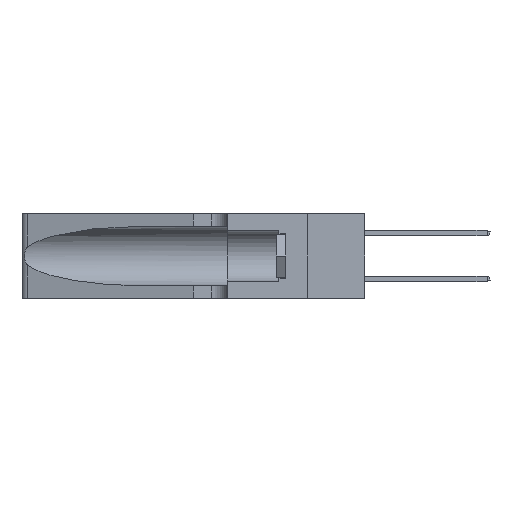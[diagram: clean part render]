
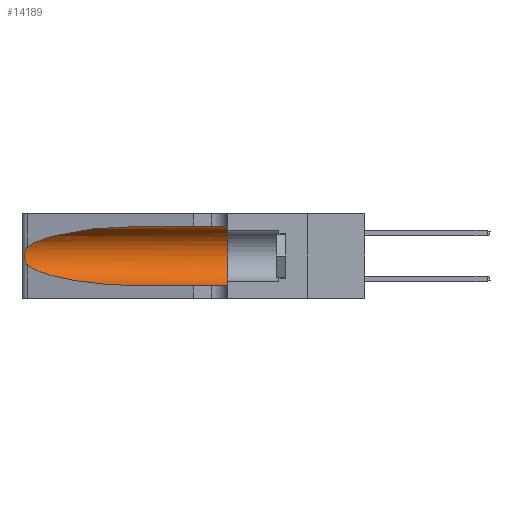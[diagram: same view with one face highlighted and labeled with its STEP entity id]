
A CAD part, left-side view. The second image highlights one B-rep face of the part: STEP entity #14189.
In plain terms, the highlighted cylindrical face has radius 3.308 mm (diameter 6.617 mm), a partial arc.
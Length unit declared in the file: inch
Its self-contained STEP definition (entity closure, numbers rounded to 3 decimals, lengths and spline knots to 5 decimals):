
#309 = CARTESIAN_POINT ( 'NONE',  ( 0.26075, 1.23896, 0.178 ) ) ;
#966 = EDGE_CURVE ( 'NONE', #5976, #19611, #1020, .T. ) ;
#1020 = LINE ( 'NONE', #4314, #5812 ) ;
#2368 = CARTESIAN_POINT ( 'NONE',  ( 0.25856, 1.23593, 0.16098 ) ) ;
#4084 = DIRECTION ( 'NONE',  ( 0., -1., 0. ) ) ;
#4173 = CARTESIAN_POINT ( 'NONE',  ( 0.25487, 1.22718, 0.22369 ) ) ;
#4314 = CARTESIAN_POINT ( 'NONE',  ( 0.1305, 1.61858, 0.05475 ) ) ;
#4342 = CARTESIAN_POINT ( 'NONE',  ( 0.25639, 1.23184, 0.21858 ) ) ;
#4435 = CARTESIAN_POINT ( 'NONE',  ( 0.25639, 1.23186, 0.15144 ) ) ;
#4637 = ORIENTED_EDGE ( 'NONE', *, *, #966, .T. ) ;
#4742 = CYLINDRICAL_SURFACE ( 'NONE', #22017, 0.13025 ) ;
#4822 = CARTESIAN_POINT ( 'NONE',  ( 0.18966, 0.96281, 0.05475 ) ) ;
#4998 = CARTESIAN_POINT ( 'NONE',  ( 0.1305, 0.35, 0.05475 ) ) ;
#5384 = EDGE_CURVE ( 'NONE', #10607, #19153, #17076, .T. ) ;
#5812 = VECTOR ( 'NONE', #4084, 39.37008 ) ;
#5912 = DIRECTION ( 'NONE',  ( 0., 0., -1. ) ) ;
#5976 = VERTEX_POINT ( 'NONE', #10400 ) ;
#6082 = AXIS2_PLACEMENT_3D ( 'NONE', #10811, #24309, #12737 ) ;
#6107 = CARTESIAN_POINT ( 'NONE',  ( 0.18966, 0.96281, 0.31525 ) ) ;
#6442 = CARTESIAN_POINT ( 'NONE',  ( 0.25487, 1.22718, 0.14631 ) ) ;
#6706 = CIRCLE ( 'NONE', #6082, 0.13025 ) ;
#6737 = CARTESIAN_POINT ( 'NONE',  ( 0.25487, 1.22718, 0.14631 ) ) ;
#8091 = VERTEX_POINT ( 'NONE', #13316 ) ;
#8113 = CARTESIAN_POINT ( 'NONE',  ( 0.1305, 0.72297, 0.31525 ) ) ;
#8356 = CARTESIAN_POINT ( 'NONE',  ( 0.25487, 1.22718, 0.22369 ) ) ;
#8822 = CARTESIAN_POINT ( 'NONE',  ( 0.25487, 1.22718, 0.22369 ) ) ;
#9886 = CARTESIAN_POINT ( 'NONE',  ( 0.1305, 1.61858, 0.185 ) ) ;
#10324 = CARTESIAN_POINT ( 'NONE',  ( 0.25854, 1.2359, 0.20912 ) ) ;
#10400 = CARTESIAN_POINT ( 'NONE',  ( 0.1305, 0.72297, 0.05475 ) ) ;
#10607 = VERTEX_POINT ( 'NONE', #8822 ) ;
#10729 =( BOUNDED_CURVE ( )  B_SPLINE_CURVE ( 3, ( #6737, #14575, #4822, #18486 ),
 .UNSPECIFIED., .F., .F. ) 
 B_SPLINE_CURVE_WITH_KNOTS ( ( 4, 4 ),
 ( 3.44316, 4.71239 ),
 .UNSPECIFIED. ) 
 CURVE ( )  GEOMETRIC_REPRESENTATION_ITEM ( )  RATIONAL_B_SPLINE_CURVE ( ( 1., 0.87, 0.87, 1. ) ) 
 REPRESENTATION_ITEM ( '' )  );
#10811 = CARTESIAN_POINT ( 'NONE',  ( 0.1305, 0.35, 0.185 ) ) ;
#10864 = VERTEX_POINT ( 'NONE', #19232 ) ;
#12256 = CARTESIAN_POINT ( 'NONE',  ( 0.26075, 1.23896, 0.19203 ) ) ;
#12737 = DIRECTION ( 'NONE',  ( 0., 0., 1. ) ) ;
#13316 = CARTESIAN_POINT ( 'NONE',  ( 0.1305, 0.72297, 0.31525 ) ) ;
#13585 = EDGE_CURVE ( 'NONE', #8091, #10607, #15205, .T. ) ;
#14188 = CARTESIAN_POINT ( 'NONE',  ( 0.26017, 1.23833, 0.17102 ) ) ;
#14189 = ADVANCED_FACE ( 'NONE', ( #20273 ), #4742, .F. ) ;
#14575 = CARTESIAN_POINT ( 'NONE',  ( 0.2373, 1.15595, 0.08982 ) ) ;
#14754 = CARTESIAN_POINT ( 'NONE',  ( 0.1305, 1.61858, 0.31525 ) ) ;
#15110 = EDGE_CURVE ( 'NONE', #19153, #5976, #10729, .T. ) ;
#15205 =( BOUNDED_CURVE ( )  B_SPLINE_CURVE ( 3, ( #8113, #6107, #15912, #4173 ),
 .UNSPECIFIED., .F., .T. ) 
 B_SPLINE_CURVE_WITH_KNOTS ( ( 4, 4 ),
 ( 1.5708, 2.84003 ),
 .UNSPECIFIED. ) 
 CURVE ( )  GEOMETRIC_REPRESENTATION_ITEM ( )  RATIONAL_B_SPLINE_CURVE ( ( 1., 0.87, 0.87, 1. ) ) 
 REPRESENTATION_ITEM ( '' )  );
#15912 = CARTESIAN_POINT ( 'NONE',  ( 0.2373, 1.15595, 0.28018 ) ) ;
#16100 = VECTOR ( 'NONE', #20565, 39.37008 ) ;
#16155 = CARTESIAN_POINT ( 'NONE',  ( 0.25789, 1.23486, 0.15765 ) ) ;
#17076 = B_SPLINE_CURVE_WITH_KNOTS ( 'NONE', 3,
 ( #8356, #18014, #4342, #21874, #10324, #23808, #12256, #309, #14188, #2368, #16155, #4435, #18101, #6442 ),
 .UNSPECIFIED., .F., .F.,
 ( 4, 2, 2, 2, 2, 2, 4 ),
 ( 0., 0.00027, 0.00053, 0.00107, 0.0016, 0.00187, 0.00214 ),
 .UNSPECIFIED. ) ;
#17082 = ORIENTED_EDGE ( 'NONE', *, *, #13585, .T. ) ;
#18014 = CARTESIAN_POINT ( 'NONE',  ( 0.25555, 1.22994, 0.2215 ) ) ;
#18027 = CARTESIAN_POINT ( 'NONE',  ( 0.25487, 1.22718, 0.14631 ) ) ;
#18101 = CARTESIAN_POINT ( 'NONE',  ( 0.25555, 1.22993, 0.14849 ) ) ;
#18486 = CARTESIAN_POINT ( 'NONE',  ( 0.1305, 0.72297, 0.05475 ) ) ;
#19153 = VERTEX_POINT ( 'NONE', #18027 ) ;
#19232 = CARTESIAN_POINT ( 'NONE',  ( 0.1305, 0.35, 0.31525 ) ) ;
#19575 = ORIENTED_EDGE ( 'NONE', *, *, #15110, .T. ) ;
#19611 = VERTEX_POINT ( 'NONE', #4998 ) ;
#19620 = EDGE_CURVE ( 'NONE', #8091, #10864, #21821, .T. ) ;
#20273 = FACE_OUTER_BOUND ( 'NONE', #21672, .T. ) ;
#20565 = DIRECTION ( 'NONE',  ( 0., -1., 0. ) ) ;
#20867 = EDGE_CURVE ( 'NONE', #10864, #19611, #6706, .T. ) ;
#20894 = ORIENTED_EDGE ( 'NONE', *, *, #19620, .F. ) ;
#21518 = ORIENTED_EDGE ( 'NONE', *, *, #20867, .F. ) ;
#21672 = EDGE_LOOP ( 'NONE', ( #17082, #22689, #19575, #4637, #21518, #20894 ) ) ;
#21821 = LINE ( 'NONE', #14754, #16100 ) ;
#21874 = CARTESIAN_POINT ( 'NONE',  ( 0.25787, 1.23484, 0.2124 ) ) ;
#22017 = AXIS2_PLACEMENT_3D ( 'NONE', #9886, #23384, #5912 ) ;
#22689 = ORIENTED_EDGE ( 'NONE', *, *, #5384, .T. ) ;
#23384 = DIRECTION ( 'NONE',  ( 0., -1., 0. ) ) ;
#23808 = CARTESIAN_POINT ( 'NONE',  ( 0.26018, 1.23835, 0.19895 ) ) ;
#24309 = DIRECTION ( 'NONE',  ( 0., 1., 0. ) ) ;
